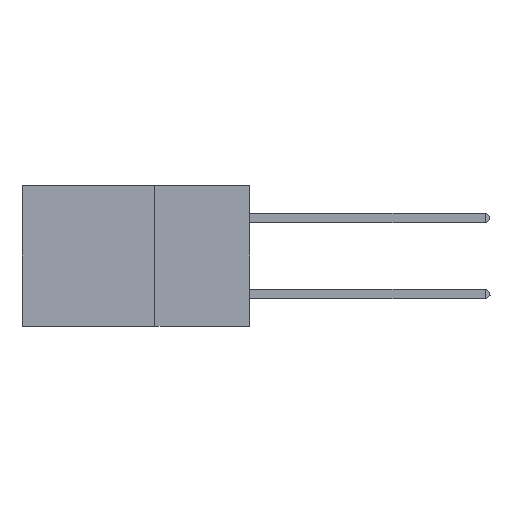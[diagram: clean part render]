
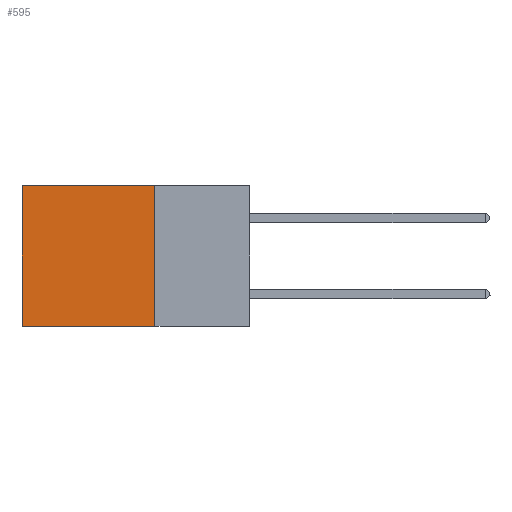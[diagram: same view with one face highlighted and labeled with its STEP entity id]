
A CAD part, left-side view. The second image highlights one B-rep face of the part: STEP entity #595.
In plain terms, the highlighted planar face has unit normal (-1, 0, 0).
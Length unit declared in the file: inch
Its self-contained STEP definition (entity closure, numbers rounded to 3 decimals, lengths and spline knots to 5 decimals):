
#173 = EDGE_CURVE ( 'NONE', #10372, #20032, #8523, .T. ) ;
#595 = ADVANCED_FACE ( 'NONE', ( #11547 ), #17408, .F. ) ;
#1354 = DIRECTION ( 'NONE',  ( 0., 1., 0. ) ) ;
#2518 = ORIENTED_EDGE ( 'NONE', *, *, #3917, .T. ) ;
#2957 = CARTESIAN_POINT ( 'NONE',  ( 0.2875, 0.6, 0. ) ) ;
#3917 = EDGE_CURVE ( 'NONE', #14078, #8668, #18893, .T. ) ;
#4252 = VECTOR ( 'NONE', #7680, 39.37008 ) ;
#4309 = CARTESIAN_POINT ( 'NONE',  ( 0.2875, 0.25, 0. ) ) ;
#4713 = CARTESIAN_POINT ( 'NONE',  ( 0.2875, 0.25, 0. ) ) ;
#5696 = DIRECTION ( 'NONE',  ( 1., 0., 0. ) ) ;
#6049 = VECTOR ( 'NONE', #1354, 39.37008 ) ;
#6320 = EDGE_LOOP ( 'NONE', ( #2518, #15824, #15204, #15694 ) ) ;
#7680 = DIRECTION ( 'NONE',  ( 0., 1., 0. ) ) ;
#8523 = LINE ( 'NONE', #4713, #15649 ) ;
#8668 = VERTEX_POINT ( 'NONE', #10435 ) ;
#9230 = CARTESIAN_POINT ( 'NONE',  ( 0.2875, 0.25, 0. ) ) ;
#9407 = EDGE_CURVE ( 'NONE', #10372, #14078, #12244, .T. ) ;
#10372 = VERTEX_POINT ( 'NONE', #4309 ) ;
#10435 = CARTESIAN_POINT ( 'NONE',  ( 0.2875, 0.6, -0.37 ) ) ;
#10859 = CARTESIAN_POINT ( 'NONE',  ( 0.2875, 0.25, -0.37 ) ) ;
#11430 = LINE ( 'NONE', #16019, #6049 ) ;
#11547 = FACE_OUTER_BOUND ( 'NONE', #6320, .T. ) ;
#11550 = DIRECTION ( 'NONE',  ( 0., 0., -1. ) ) ;
#12244 = LINE ( 'NONE', #12667, #4252 ) ;
#12667 = CARTESIAN_POINT ( 'NONE',  ( 0.2875, 0.25, 0. ) ) ;
#12934 = DIRECTION ( 'NONE',  ( 0., 0., -1. ) ) ;
#14078 = VERTEX_POINT ( 'NONE', #2957 ) ;
#15204 = ORIENTED_EDGE ( 'NONE', *, *, #173, .F. ) ;
#15620 = DIRECTION ( 'NONE',  ( 0., 0., -1. ) ) ;
#15649 = VECTOR ( 'NONE', #12934, 39.37008 ) ;
#15694 = ORIENTED_EDGE ( 'NONE', *, *, #9407, .T. ) ;
#15824 = ORIENTED_EDGE ( 'NONE', *, *, #17355, .F. ) ;
#16019 = CARTESIAN_POINT ( 'NONE',  ( 0.2875, 0.25, -0.37 ) ) ;
#16668 = AXIS2_PLACEMENT_3D ( 'NONE', #9230, #5696, #15620 ) ;
#16806 = VECTOR ( 'NONE', #11550, 39.37008 ) ;
#17355 = EDGE_CURVE ( 'NONE', #20032, #8668, #11430, .T. ) ;
#17408 = PLANE ( 'NONE',  #16668 ) ;
#18893 = LINE ( 'NONE', #19091, #16806 ) ;
#19091 = CARTESIAN_POINT ( 'NONE',  ( 0.2875, 0.6, 0. ) ) ;
#20032 = VERTEX_POINT ( 'NONE', #10859 ) ;
